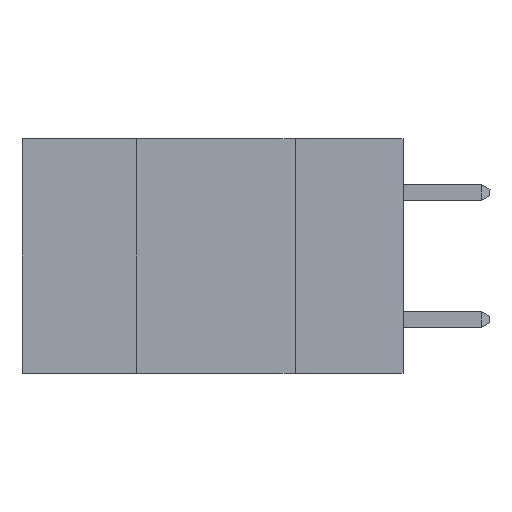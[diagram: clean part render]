
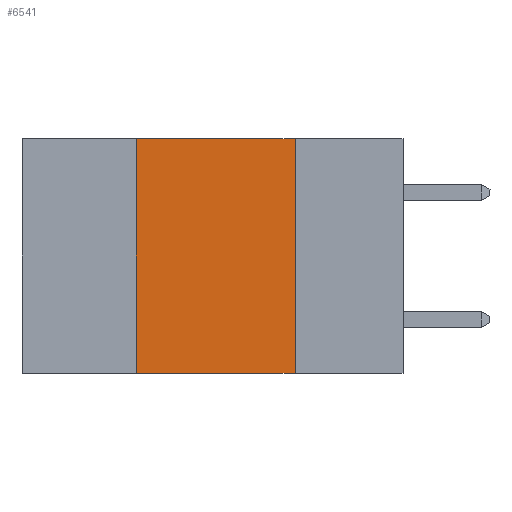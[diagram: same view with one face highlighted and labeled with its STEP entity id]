
A CAD part, left-side view. The second image highlights one B-rep face of the part: STEP entity #6541.
In plain terms, the highlighted planar face has unit normal (-1, 0, 0).
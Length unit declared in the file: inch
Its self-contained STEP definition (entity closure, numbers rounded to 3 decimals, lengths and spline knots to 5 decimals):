
#17 = ORIENTED_EDGE ( 'NONE', *, *, #3864, .F. ) ;
#117 = EDGE_CURVE ( 'NONE', #5810, #3134, #13051, .T. ) ;
#258 = VECTOR ( 'NONE', #1032, 39.37008 ) ;
#390 = VERTEX_POINT ( 'NONE', #920 ) ;
#588 = LINE ( 'NONE', #8365, #258 ) ;
#920 = CARTESIAN_POINT ( 'NONE',  ( 0., 0.17, 0. ) ) ;
#955 = DIRECTION ( 'NONE',  ( 0., 0., 1. ) ) ;
#1032 = DIRECTION ( 'NONE',  ( 0., 0., -1. ) ) ;
#1230 = CARTESIAN_POINT ( 'NONE',  ( 0., 0.42, 0. ) ) ;
#1679 = DIRECTION ( 'NONE',  ( 0., -1., 0. ) ) ;
#1728 = CARTESIAN_POINT ( 'NONE',  ( 0., 0.6, -0.37 ) ) ;
#1792 = EDGE_CURVE ( 'NONE', #5810, #2135, #10042, .T. ) ;
#2135 = VERTEX_POINT ( 'NONE', #6451 ) ;
#2559 = EDGE_LOOP ( 'NONE', ( #5353, #17, #11258, #8789 ) ) ;
#2811 = DIRECTION ( 'NONE',  ( 0., -1., 0. ) ) ;
#3058 = LINE ( 'NONE', #9117, #5559 ) ;
#3134 = VERTEX_POINT ( 'NONE', #9135 ) ;
#3416 = EDGE_CURVE ( 'NONE', #390, #2135, #588, .T. ) ;
#3864 = EDGE_CURVE ( 'NONE', #3134, #390, #3058, .T. ) ;
#5353 = ORIENTED_EDGE ( 'NONE', *, *, #3416, .F. ) ;
#5559 = VECTOR ( 'NONE', #2811, 39.37008 ) ;
#5810 = VERTEX_POINT ( 'NONE', #8800 ) ;
#5940 = DIRECTION ( 'NONE',  ( 0., 0., -1. ) ) ;
#6451 = CARTESIAN_POINT ( 'NONE',  ( 0., 0.17, -0.37 ) ) ;
#6541 = ADVANCED_FACE ( 'NONE', ( #12250 ), #11177, .F. ) ;
#6958 = CARTESIAN_POINT ( 'NONE',  ( 0., 0.6, 0. ) ) ;
#7593 = VECTOR ( 'NONE', #955, 39.37008 ) ;
#7711 = AXIS2_PLACEMENT_3D ( 'NONE', #6958, #12188, #5940 ) ;
#8365 = CARTESIAN_POINT ( 'NONE',  ( 0., 0.17, 0. ) ) ;
#8789 = ORIENTED_EDGE ( 'NONE', *, *, #1792, .T. ) ;
#8800 = CARTESIAN_POINT ( 'NONE',  ( 0., 0.42, -0.37 ) ) ;
#9117 = CARTESIAN_POINT ( 'NONE',  ( 0., 0.6, 0. ) ) ;
#9135 = CARTESIAN_POINT ( 'NONE',  ( 0., 0.42, 0. ) ) ;
#10042 = LINE ( 'NONE', #1728, #12738 ) ;
#11177 = PLANE ( 'NONE',  #7711 ) ;
#11258 = ORIENTED_EDGE ( 'NONE', *, *, #117, .F. ) ;
#12188 = DIRECTION ( 'NONE',  ( 1., 0., 0. ) ) ;
#12250 = FACE_OUTER_BOUND ( 'NONE', #2559, .T. ) ;
#12738 = VECTOR ( 'NONE', #1679, 39.37008 ) ;
#13051 = LINE ( 'NONE', #1230, #7593 ) ;
